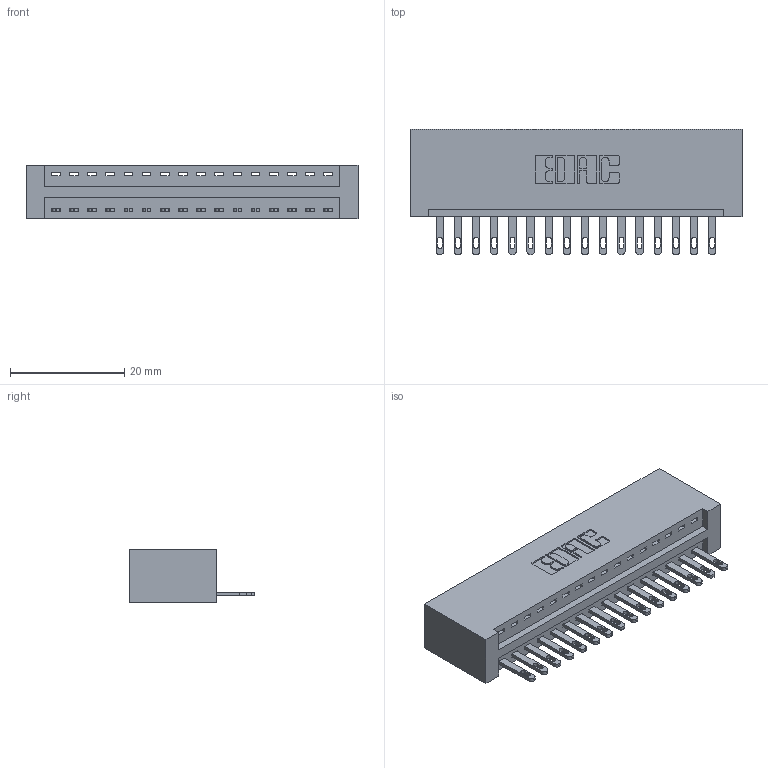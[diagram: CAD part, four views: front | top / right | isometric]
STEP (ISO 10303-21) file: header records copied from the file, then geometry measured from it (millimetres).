
FILE_DESCRIPTION (( 'STEP AP203' ), '1' );
FILE_NAME ('346-016-500-101.STEP', '2018-08-20T03:16:33', ( '' ), ( '' ), 'SwSTEP 2.0', 'SolidWorks 2016', '' );
FILE_SCHEMA (( 'CONFIG_CONTROL_DESIGN' ));
Length unit declared in the file: inch
Products named in the file (3): 346 Part_No Mounting Lugs; 345-292-001_345-293-100; 346-016-500-101
Assembly tree (17 placements, depth 2):
  346-016-500-101
    346 Part_No Mounting Lugs
    345-292-001_345-293-100  x16
Bounding box: 58.04 x 21.84 x 9.4 mm (x, y, z)
Volume: 5935.8 mm3; surface area: 7250.8 mm2
Topology: 17 solids, 17 shells, 978 faces, 2993 edges, 1994 vertices
Faces by surface type: plane 616, cylinder 362
Entity records: 13083 total; most frequent: CARTESIAN_POINT 2256, ORIENTED_EDGE 2206, DIRECTION 2019, EDGE_CURVE 1103, VECTOR 911, LINE 911, VERTEX_POINT 734, AXIS2_PLACEMENT_3D 554
